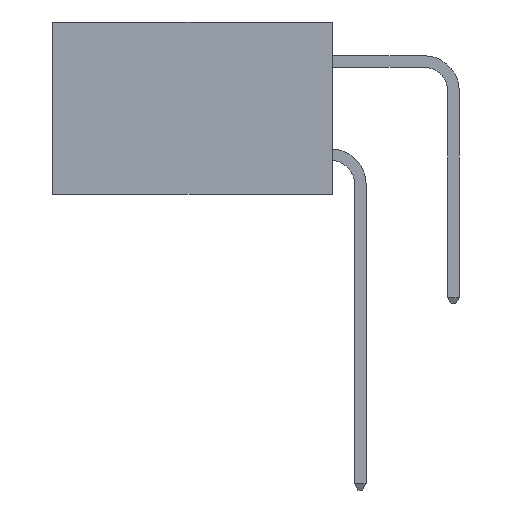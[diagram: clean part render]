
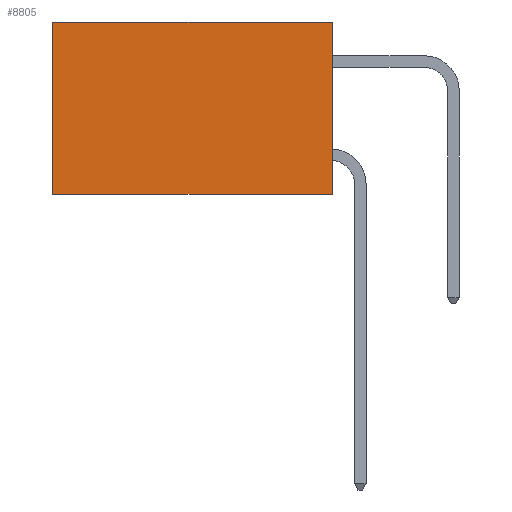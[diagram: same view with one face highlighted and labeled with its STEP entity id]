
A CAD part, left-side view. The second image highlights one B-rep face of the part: STEP entity #8805.
In plain terms, the highlighted planar face has unit normal (-1, 0, 0).
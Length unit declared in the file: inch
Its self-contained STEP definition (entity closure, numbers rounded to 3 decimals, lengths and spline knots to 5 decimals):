
#1631 = VERTEX_POINT ( 'NONE', #16550 ) ;
#1882 = DIRECTION ( 'NONE',  ( 0., 1., 0. ) ) ;
#1958 = CARTESIAN_POINT ( 'NONE',  ( 0.298, 0., 0. ) ) ;
#1965 = CARTESIAN_POINT ( 'NONE',  ( 0.298, 0.6, -0.37 ) ) ;
#2958 = EDGE_CURVE ( 'NONE', #1631, #8894, #6058, .T. ) ;
#5356 = AXIS2_PLACEMENT_3D ( 'NONE', #20060, #21860, #10862 ) ;
#5617 = CARTESIAN_POINT ( 'NONE',  ( 0.298, 0.6, 0. ) ) ;
#5791 = ORIENTED_EDGE ( 'NONE', *, *, #17535, .F. ) ;
#6058 = LINE ( 'NONE', #1958, #19045 ) ;
#6477 = DIRECTION ( 'NONE',  ( 0., 0., -1. ) ) ;
#6828 = CARTESIAN_POINT ( 'NONE',  ( 0.298, 0., -0.37 ) ) ;
#7499 = VECTOR ( 'NONE', #6477, 39.37008 ) ;
#7593 = FACE_OUTER_BOUND ( 'NONE', #19121, .T. ) ;
#8805 = ADVANCED_FACE ( 'NONE', ( #7593 ), #9028, .F. ) ;
#8894 = VERTEX_POINT ( 'NONE', #5617 ) ;
#9028 = PLANE ( 'NONE',  #5356 ) ;
#10234 = EDGE_CURVE ( 'NONE', #8894, #20538, #18750, .T. ) ;
#10422 = DIRECTION ( 'NONE',  ( 0., 1., 0. ) ) ;
#10862 = DIRECTION ( 'NONE',  ( 0., 0., -1. ) ) ;
#12184 = ORIENTED_EDGE ( 'NONE', *, *, #10234, .T. ) ;
#12306 = ORIENTED_EDGE ( 'NONE', *, *, #2958, .T. ) ;
#15517 = LINE ( 'NONE', #15966, #23478 ) ;
#15966 = CARTESIAN_POINT ( 'NONE',  ( 0.298, 0., -0.37 ) ) ;
#16258 = ORIENTED_EDGE ( 'NONE', *, *, #22132, .F. ) ;
#16550 = CARTESIAN_POINT ( 'NONE',  ( 0.298, 0., 0. ) ) ;
#16600 = DIRECTION ( 'NONE',  ( 0., 0., -1. ) ) ;
#17535 = EDGE_CURVE ( 'NONE', #1631, #18856, #17880, .T. ) ;
#17880 = LINE ( 'NONE', #22981, #7499 ) ;
#18513 = VECTOR ( 'NONE', #16600, 39.37008 ) ;
#18750 = LINE ( 'NONE', #20235, #18513 ) ;
#18856 = VERTEX_POINT ( 'NONE', #6828 ) ;
#19045 = VECTOR ( 'NONE', #1882, 39.37008 ) ;
#19121 = EDGE_LOOP ( 'NONE', ( #12184, #16258, #5791, #12306 ) ) ;
#20060 = CARTESIAN_POINT ( 'NONE',  ( 0.298, 0., 0. ) ) ;
#20235 = CARTESIAN_POINT ( 'NONE',  ( 0.298, 0.6, 0. ) ) ;
#20538 = VERTEX_POINT ( 'NONE', #1965 ) ;
#21860 = DIRECTION ( 'NONE',  ( 1., 0., 0. ) ) ;
#22132 = EDGE_CURVE ( 'NONE', #18856, #20538, #15517, .T. ) ;
#22981 = CARTESIAN_POINT ( 'NONE',  ( 0.298, 0., 0. ) ) ;
#23478 = VECTOR ( 'NONE', #10422, 39.37008 ) ;
